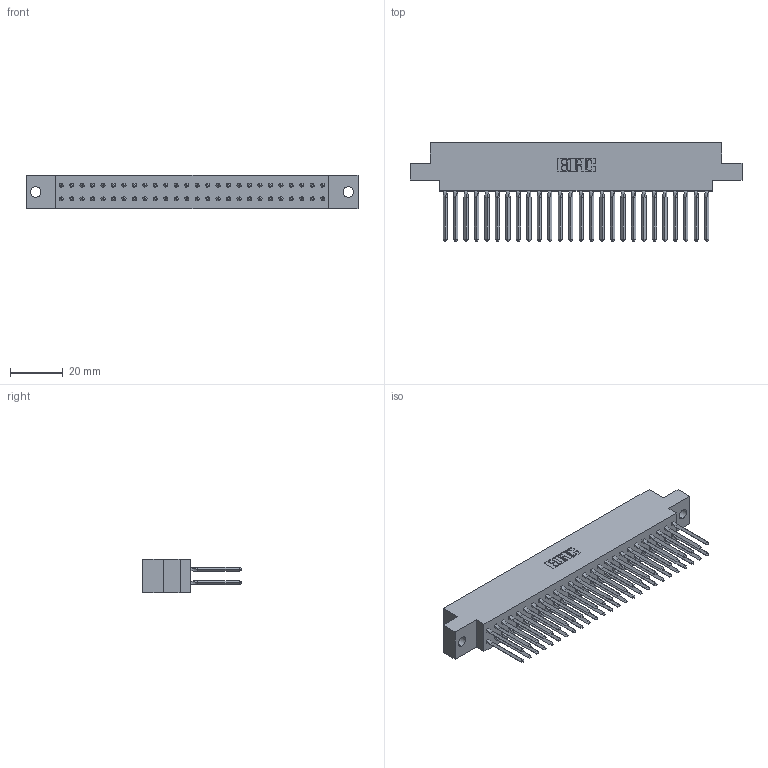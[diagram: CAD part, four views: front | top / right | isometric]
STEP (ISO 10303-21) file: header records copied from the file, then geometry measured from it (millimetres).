
FILE_DESCRIPTION (( 'STEP AP203' ), '1' );
FILE_NAME ('317-052-542-804.STEP', '2020-02-28T03:34:34', ( '' ), ( '' ), 'SwSTEP 2.0', 'SolidWorks 2016', '' );
FILE_SCHEMA (( 'CONFIG_CONTROL_DESIGN' ));
Length unit declared in the file: inch
Products named in the file (3): 317-290-003_542; 317 Part_.156 Dia - TH; 317-052-542-804
Assembly tree (53 placements, depth 2):
  317-052-542-804
    317 Part_.156 Dia - TH
    317-290-003_542  x52
Bounding box: 125.73 x 37.34 x 12.7 mm (x, y, z)
Volume: 19994.4 mm3; surface area: 27107.7 mm2
Topology: 53 solids, 53 shells, 3066 faces, 8595 edges, 5486 vertices
Faces by surface type: plane 2450, cylinder 408, bspline 208
Entity records: 38835 total; most frequent: CARTESIAN_POINT 7021, ORIENTED_EDGE 6684, DIRECTION 5650, EDGE_CURVE 3342, LINE 3172, VECTOR 3172, VERTEX_POINT 2222, AXIS2_PLACEMENT_3D 1239
